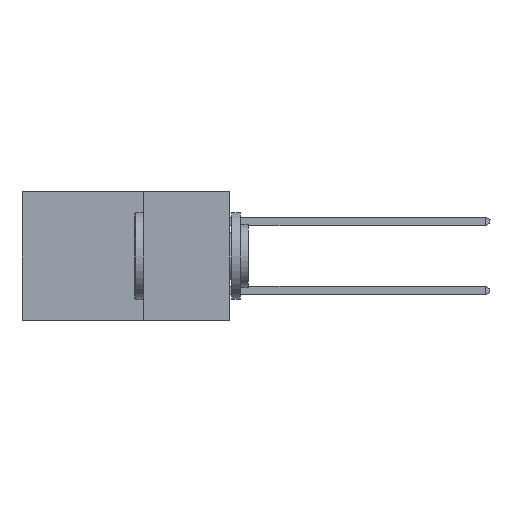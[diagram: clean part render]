
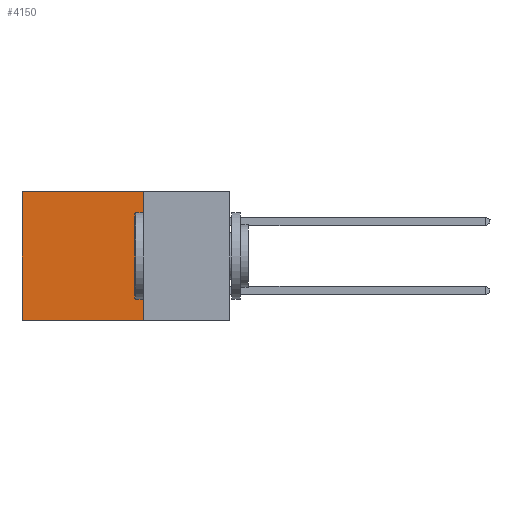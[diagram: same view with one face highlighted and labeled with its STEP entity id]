
A CAD part, left-side view. The second image highlights one B-rep face of the part: STEP entity #4150.
In plain terms, the highlighted planar face has unit normal (-1, 0, 0).
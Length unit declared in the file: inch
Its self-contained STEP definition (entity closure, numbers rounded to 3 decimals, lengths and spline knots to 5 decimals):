
#1172 = DIRECTION ( 'NONE',  ( 0., 0., -1. ) ) ;
#1368 = CARTESIAN_POINT ( 'NONE',  ( 0.2615, 0.25, 0. ) ) ;
#1658 = EDGE_CURVE ( 'NONE', #3739, #1680, #13133, .T. ) ;
#1680 = VERTEX_POINT ( 'NONE', #6133 ) ;
#2746 = LINE ( 'NONE', #7166, #4074 ) ;
#2858 = CARTESIAN_POINT ( 'NONE',  ( 0.2615, 0.25, -0.37 ) ) ;
#3739 = VERTEX_POINT ( 'NONE', #17344 ) ;
#4009 = DIRECTION ( 'NONE',  ( 0., 1., 0. ) ) ;
#4074 = VECTOR ( 'NONE', #16883, 39.37008 ) ;
#4150 = ADVANCED_FACE ( 'NONE', ( #14123 ), #6232, .F. ) ;
#5110 = LINE ( 'NONE', #9552, #14072 ) ;
#5188 = VERTEX_POINT ( 'NONE', #1368 ) ;
#6133 = CARTESIAN_POINT ( 'NONE',  ( 0.2615, 0.6, -0.37 ) ) ;
#6232 = PLANE ( 'NONE',  #8733 ) ;
#7166 = CARTESIAN_POINT ( 'NONE',  ( 0.2615, 0.25, -0.37 ) ) ;
#8250 = ORIENTED_EDGE ( 'NONE', *, *, #1658, .T. ) ;
#8733 = AXIS2_PLACEMENT_3D ( 'NONE', #2858, #8960, #1172 ) ;
#8960 = DIRECTION ( 'NONE',  ( 1., 0., 0. ) ) ;
#9552 = CARTESIAN_POINT ( 'NONE',  ( 0.2615, 0.25, -0.37 ) ) ;
#10154 = EDGE_CURVE ( 'NONE', #5188, #3739, #12023, .T. ) ;
#11143 = ORIENTED_EDGE ( 'NONE', *, *, #10154, .T. ) ;
#11447 = ORIENTED_EDGE ( 'NONE', *, *, #16017, .F. ) ;
#11707 = EDGE_LOOP ( 'NONE', ( #8250, #16833, #11447, #11143 ) ) ;
#11772 = VERTEX_POINT ( 'NONE', #15823 ) ;
#12023 = LINE ( 'NONE', #18456, #18089 ) ;
#12808 = EDGE_CURVE ( 'NONE', #11772, #1680, #5110, .T. ) ;
#12924 = DIRECTION ( 'NONE',  ( 0., 1., 0. ) ) ;
#13133 = LINE ( 'NONE', #18000, #18314 ) ;
#14072 = VECTOR ( 'NONE', #12924, 39.37008 ) ;
#14123 = FACE_OUTER_BOUND ( 'NONE', #11707, .T. ) ;
#14606 = DIRECTION ( 'NONE',  ( 0., 0., -1. ) ) ;
#15823 = CARTESIAN_POINT ( 'NONE',  ( 0.2615, 0.25, -0.37 ) ) ;
#16017 = EDGE_CURVE ( 'NONE', #5188, #11772, #2746, .T. ) ;
#16833 = ORIENTED_EDGE ( 'NONE', *, *, #12808, .F. ) ;
#16883 = DIRECTION ( 'NONE',  ( 0., 0., -1. ) ) ;
#17344 = CARTESIAN_POINT ( 'NONE',  ( 0.2615, 0.6, 0. ) ) ;
#18000 = CARTESIAN_POINT ( 'NONE',  ( 0.2615, 0.6, -0.37 ) ) ;
#18089 = VECTOR ( 'NONE', #4009, 39.37008 ) ;
#18314 = VECTOR ( 'NONE', #14606, 39.37008 ) ;
#18456 = CARTESIAN_POINT ( 'NONE',  ( 0.2615, 0.25, 0. ) ) ;
